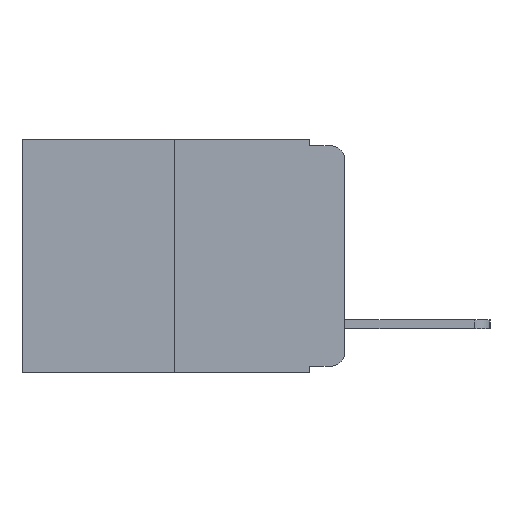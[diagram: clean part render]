
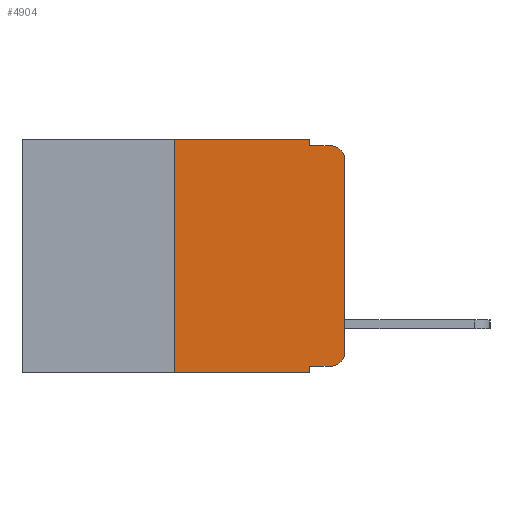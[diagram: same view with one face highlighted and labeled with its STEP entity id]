
A CAD part, left-side view. The second image highlights one B-rep face of the part: STEP entity #4904.
In plain terms, the highlighted planar face has unit normal (-1, 0, 0).
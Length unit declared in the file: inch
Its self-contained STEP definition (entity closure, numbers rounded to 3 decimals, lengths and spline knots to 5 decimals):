
#65 = VERTEX_POINT ( 'NONE', #7113 ) ;
#223 = EDGE_LOOP ( 'NONE', ( #5749, #10268, #1653, #975, #3385, #3572, #3246, #11408, #2651, #7000 ) ) ;
#244 = VECTOR ( 'NONE', #4600, 39.37008 ) ;
#784 = CARTESIAN_POINT ( 'NONE',  ( 0., 0.473, 0. ) ) ;
#840 = VERTEX_POINT ( 'NONE', #9573 ) ;
#975 = ORIENTED_EDGE ( 'NONE', *, *, #1240, .F. ) ;
#1114 = VECTOR ( 'NONE', #6214, 39.37008 ) ;
#1144 = VERTEX_POINT ( 'NONE', #1179 ) ;
#1166 = EDGE_CURVE ( 'NONE', #1903, #11553, #11550, .T. ) ;
#1179 = CARTESIAN_POINT ( 'NONE',  ( 0., 0.051, -0.333 ) ) ;
#1182 = EDGE_CURVE ( 'NONE', #11553, #840, #7297, .T. ) ;
#1225 = EDGE_CURVE ( 'NONE', #3038, #840, #6752, .T. ) ;
#1240 = EDGE_CURVE ( 'NONE', #10605, #3038, #3835, .T. ) ;
#1269 = DIRECTION ( 'NONE',  ( 0., -1., 0. ) ) ;
#1305 = EDGE_CURVE ( 'NONE', #2425, #5607, #2836, .T. ) ;
#1328 = EDGE_CURVE ( 'NONE', #1144, #65, #7718, .T. ) ;
#1333 = CARTESIAN_POINT ( 'NONE',  ( 0., 0.25, -0.343 ) ) ;
#1344 = EDGE_CURVE ( 'NONE', #1144, #7354, #2206, .T. ) ;
#1382 = EDGE_CURVE ( 'NONE', #7354, #1903, #9636, .T. ) ;
#1406 = CARTESIAN_POINT ( 'NONE',  ( 0., 0.051, -0.333 ) ) ;
#1653 = ORIENTED_EDGE ( 'NONE', *, *, #1225, .F. ) ;
#1790 = FACE_OUTER_BOUND ( 'NONE', #223, .T. ) ;
#1853 = CARTESIAN_POINT ( 'NONE',  ( 0., 0., 0. ) ) ;
#1903 = VERTEX_POINT ( 'NONE', #8085 ) ;
#1909 = DIRECTION ( 'NONE',  ( 0., 0., -1. ) ) ;
#2206 = LINE ( 'NONE', #1406, #9385 ) ;
#2237 = CARTESIAN_POINT ( 'NONE',  ( 0., 0.02, -0.333 ) ) ;
#2425 = VERTEX_POINT ( 'NONE', #1333 ) ;
#2504 = LINE ( 'NONE', #784, #11640 ) ;
#2651 = ORIENTED_EDGE ( 'NONE', *, *, #1344, .T. ) ;
#2836 = LINE ( 'NONE', #9980, #5297 ) ;
#3038 = VERTEX_POINT ( 'NONE', #6019 ) ;
#3089 = PLANE ( 'NONE',  #11696 ) ;
#3240 = DIRECTION ( 'NONE',  ( 0., -1., 0. ) ) ;
#3246 = ORIENTED_EDGE ( 'NONE', *, *, #10696, .T. ) ;
#3319 = DIRECTION ( 'NONE',  ( 0., 0., 1. ) ) ;
#3373 = DIRECTION ( 'NONE',  ( 0., 0., 1. ) ) ;
#3385 = ORIENTED_EDGE ( 'NONE', *, *, #10192, .F. ) ;
#3572 = ORIENTED_EDGE ( 'NONE', *, *, #1305, .F. ) ;
#3618 = CARTESIAN_POINT ( 'NONE',  ( 0., 0.02, -0.313 ) ) ;
#3651 = DIRECTION ( 'NONE',  ( 0., 0., -1. ) ) ;
#3718 = DIRECTION ( 'NONE',  ( -1., 0., 0. ) ) ;
#3835 = LINE ( 'NONE', #10839, #4175 ) ;
#4175 = VECTOR ( 'NONE', #6607, 39.37008 ) ;
#4600 = DIRECTION ( 'NONE',  ( 0., -1., 0. ) ) ;
#4904 = ADVANCED_FACE ( 'NONE', ( #1790 ), #3089, .F. ) ;
#4986 = VECTOR ( 'NONE', #7659, 39.37008 ) ;
#5297 = VECTOR ( 'NONE', #3373, 39.37008 ) ;
#5607 = VERTEX_POINT ( 'NONE', #6339 ) ;
#5749 = ORIENTED_EDGE ( 'NONE', *, *, #1166, .T. ) ;
#5855 = CARTESIAN_POINT ( 'NONE',  ( 0., 0., -0.03 ) ) ;
#6019 = CARTESIAN_POINT ( 'NONE',  ( 0., 0.051, -0.01 ) ) ;
#6214 = DIRECTION ( 'NONE',  ( 0., -1., 0. ) ) ;
#6292 = CARTESIAN_POINT ( 'NONE',  ( 0., 0.051, 0. ) ) ;
#6339 = CARTESIAN_POINT ( 'NONE',  ( 0., 0.25, 0. ) ) ;
#6607 = DIRECTION ( 'NONE',  ( 0., 0., -1. ) ) ;
#6752 = LINE ( 'NONE', #11136, #1114 ) ;
#7000 = ORIENTED_EDGE ( 'NONE', *, *, #1382, .T. ) ;
#7113 = CARTESIAN_POINT ( 'NONE',  ( 0., 0.051, -0.343 ) ) ;
#7297 = CIRCLE ( 'NONE', #11172, 0.02 ) ;
#7354 = VERTEX_POINT ( 'NONE', #2237 ) ;
#7659 = DIRECTION ( 'NONE',  ( 0., 0., -1. ) ) ;
#7718 = LINE ( 'NONE', #6292, #4986 ) ;
#7760 = DIRECTION ( 'NONE',  ( 1., 0., 0. ) ) ;
#8085 = CARTESIAN_POINT ( 'NONE',  ( 0., 0., -0.313 ) ) ;
#8386 = LINE ( 'NONE', #9059, #244 ) ;
#9003 = DIRECTION ( 'NONE',  ( 0., 0., -1. ) ) ;
#9059 = CARTESIAN_POINT ( 'NONE',  ( 0., 0.473, -0.343 ) ) ;
#9265 = VECTOR ( 'NONE', #3319, 39.37008 ) ;
#9385 = VECTOR ( 'NONE', #1269, 39.37008 ) ;
#9573 = CARTESIAN_POINT ( 'NONE',  ( 0., 0.02, -0.01 ) ) ;
#9636 = CIRCLE ( 'NONE', #10917, 0.02 ) ;
#9980 = CARTESIAN_POINT ( 'NONE',  ( 0., 0.25, 0. ) ) ;
#10192 = EDGE_CURVE ( 'NONE', #5607, #10605, #2504, .T. ) ;
#10268 = ORIENTED_EDGE ( 'NONE', *, *, #1182, .T. ) ;
#10605 = VERTEX_POINT ( 'NONE', #11309 ) ;
#10696 = EDGE_CURVE ( 'NONE', #2425, #65, #8386, .T. ) ;
#10839 = CARTESIAN_POINT ( 'NONE',  ( 0., 0.051, 0. ) ) ;
#10917 = AXIS2_PLACEMENT_3D ( 'NONE', #3618, #3718, #3651 ) ;
#11136 = CARTESIAN_POINT ( 'NONE',  ( 0., 0.051, -0.01 ) ) ;
#11172 = AXIS2_PLACEMENT_3D ( 'NONE', #11341, #11236, #9003 ) ;
#11236 = DIRECTION ( 'NONE',  ( -1., 0., 0. ) ) ;
#11244 = CARTESIAN_POINT ( 'NONE',  ( 0., 0.473, 0. ) ) ;
#11309 = CARTESIAN_POINT ( 'NONE',  ( 0., 0.051, 0. ) ) ;
#11341 = CARTESIAN_POINT ( 'NONE',  ( 0., 0.02, -0.03 ) ) ;
#11408 = ORIENTED_EDGE ( 'NONE', *, *, #1328, .F. ) ;
#11550 = LINE ( 'NONE', #1853, #9265 ) ;
#11553 = VERTEX_POINT ( 'NONE', #5855 ) ;
#11640 = VECTOR ( 'NONE', #3240, 39.37008 ) ;
#11696 = AXIS2_PLACEMENT_3D ( 'NONE', #11244, #7760, #1909 ) ;
